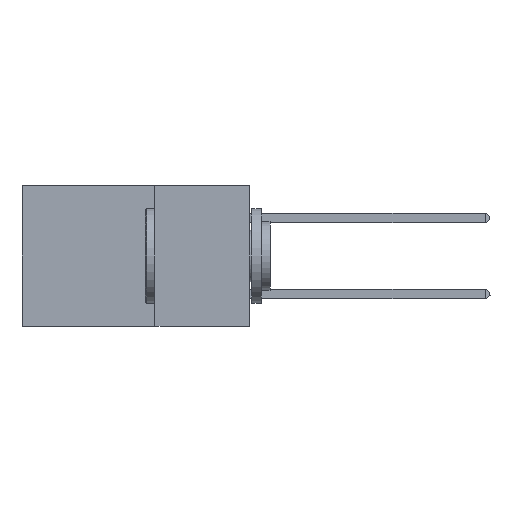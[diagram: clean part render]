
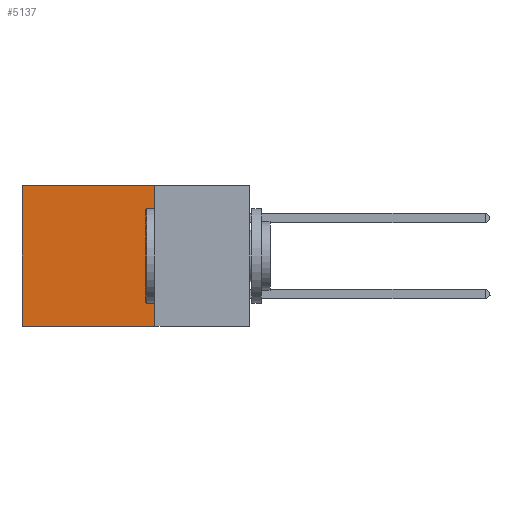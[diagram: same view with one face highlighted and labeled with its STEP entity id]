
A CAD part, left-side view. The second image highlights one B-rep face of the part: STEP entity #5137.
In plain terms, the highlighted planar face has unit normal (-1, 0, 0).
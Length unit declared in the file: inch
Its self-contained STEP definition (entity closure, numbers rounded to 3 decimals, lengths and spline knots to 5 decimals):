
#50 = ORIENTED_EDGE ( 'NONE', *, *, #10320, .T. ) ;
#602 = CARTESIAN_POINT ( 'NONE',  ( 0.2875, 0.25, 0. ) ) ;
#677 = VERTEX_POINT ( 'NONE', #9576 ) ;
#1093 = LINE ( 'NONE', #13227, #9129 ) ;
#1473 = CARTESIAN_POINT ( 'NONE',  ( 0.2875, 0.25, 0. ) ) ;
#1734 = EDGE_LOOP ( 'NONE', ( #50, #3079, #8549, #3433 ) ) ;
#1896 = VERTEX_POINT ( 'NONE', #7117 ) ;
#1968 = FACE_OUTER_BOUND ( 'NONE', #1734, .T. ) ;
#2176 = EDGE_CURVE ( 'NONE', #13128, #677, #11450, .T. ) ;
#2503 = VERTEX_POINT ( 'NONE', #12519 ) ;
#2622 = DIRECTION ( 'NONE',  ( 1., 0., 0. ) ) ;
#2661 = LINE ( 'NONE', #9764, #13179 ) ;
#3079 = ORIENTED_EDGE ( 'NONE', *, *, #6381, .F. ) ;
#3433 = ORIENTED_EDGE ( 'NONE', *, *, #4706, .T. ) ;
#4706 = EDGE_CURVE ( 'NONE', #13128, #1896, #1093, .T. ) ;
#5137 = ADVANCED_FACE ( 'NONE', ( #1968 ), #7763, .F. ) ;
#5422 = CARTESIAN_POINT ( 'NONE',  ( 0.2875, 0.6, 0. ) ) ;
#5430 = VECTOR ( 'NONE', #9980, 39.37008 ) ;
#5695 = LINE ( 'NONE', #5422, #6008 ) ;
#6008 = VECTOR ( 'NONE', #13464, 39.37008 ) ;
#6381 = EDGE_CURVE ( 'NONE', #677, #2503, #2661, .T. ) ;
#7117 = CARTESIAN_POINT ( 'NONE',  ( 0.2875, 0.6, 0. ) ) ;
#7223 = DIRECTION ( 'NONE',  ( 0., 1., 0. ) ) ;
#7437 = AXIS2_PLACEMENT_3D ( 'NONE', #1473, #2622, #9791 ) ;
#7763 = PLANE ( 'NONE',  #7437 ) ;
#8549 = ORIENTED_EDGE ( 'NONE', *, *, #2176, .F. ) ;
#9115 = CARTESIAN_POINT ( 'NONE',  ( 0.2875, 0.25, 0. ) ) ;
#9129 = VECTOR ( 'NONE', #7223, 39.37008 ) ;
#9576 = CARTESIAN_POINT ( 'NONE',  ( 0.2875, 0.25, -0.37 ) ) ;
#9764 = CARTESIAN_POINT ( 'NONE',  ( 0.2875, 0.25, -0.37 ) ) ;
#9791 = DIRECTION ( 'NONE',  ( 0., 0., -1. ) ) ;
#9980 = DIRECTION ( 'NONE',  ( 0., 0., -1. ) ) ;
#10320 = EDGE_CURVE ( 'NONE', #1896, #2503, #5695, .T. ) ;
#11450 = LINE ( 'NONE', #9115, #5430 ) ;
#11821 = DIRECTION ( 'NONE',  ( 0., 1., 0. ) ) ;
#12519 = CARTESIAN_POINT ( 'NONE',  ( 0.2875, 0.6, -0.37 ) ) ;
#13128 = VERTEX_POINT ( 'NONE', #602 ) ;
#13179 = VECTOR ( 'NONE', #11821, 39.37008 ) ;
#13227 = CARTESIAN_POINT ( 'NONE',  ( 0.2875, 0.25, 0. ) ) ;
#13464 = DIRECTION ( 'NONE',  ( 0., 0., -1. ) ) ;
